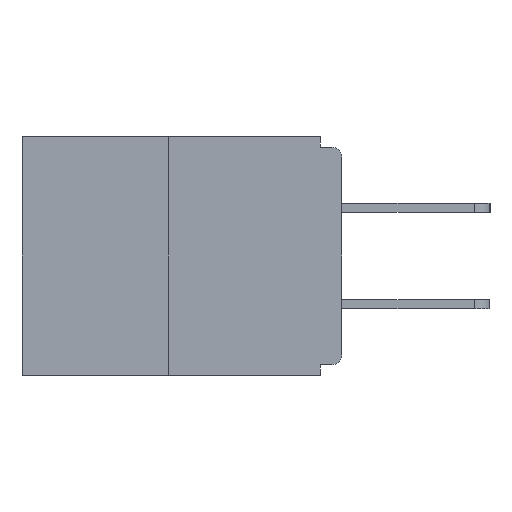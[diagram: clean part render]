
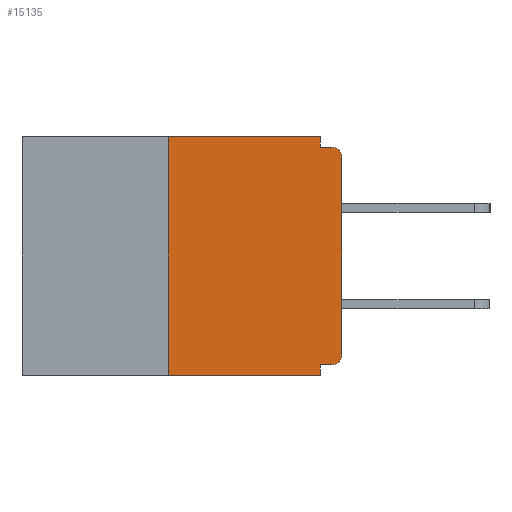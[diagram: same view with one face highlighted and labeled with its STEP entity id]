
A CAD part, left-side view. The second image highlights one B-rep face of the part: STEP entity #15135.
In plain terms, the highlighted planar face has unit normal (-1, 0, 0).
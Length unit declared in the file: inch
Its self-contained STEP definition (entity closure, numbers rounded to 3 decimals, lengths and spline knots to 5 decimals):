
#8 = CARTESIAN_POINT ( 'NONE',  ( 0., 0.015, -0.015 ) ) ;
#1059 = CARTESIAN_POINT ( 'NONE',  ( 0., 0.015, -0.03 ) ) ;
#1124 = CARTESIAN_POINT ( 'NONE',  ( 0., 0.015, -0.313 ) ) ;
#1439 = CARTESIAN_POINT ( 'NONE',  ( 0., 0., 0. ) ) ;
#1469 = VERTEX_POINT ( 'NONE', #16318 ) ;
#2100 = DIRECTION ( 'NONE',  ( 0., 0., -1. ) ) ;
#2277 = EDGE_LOOP ( 'NONE', ( #11711, #16246, #13082, #7259, #3381, #3264, #10527, #13912, #7482, #14920 ) ) ;
#2496 = EDGE_CURVE ( 'NONE', #3343, #14005, #4907, .T. ) ;
#2939 = LINE ( 'NONE', #13357, #13848 ) ;
#3190 = VECTOR ( 'NONE', #5323, 39.37008 ) ;
#3264 = ORIENTED_EDGE ( 'NONE', *, *, #3744, .T. ) ;
#3283 = EDGE_CURVE ( 'NONE', #13364, #11104, #16549, .T. ) ;
#3343 = VERTEX_POINT ( 'NONE', #10244 ) ;
#3381 = ORIENTED_EDGE ( 'NONE', *, *, #13331, .F. ) ;
#3552 = CARTESIAN_POINT ( 'NONE',  ( 0., 0.46, -0.343 ) ) ;
#3625 = DIRECTION ( 'NONE',  ( 0., 0., -1. ) ) ;
#3744 = EDGE_CURVE ( 'NONE', #7836, #12753, #15659, .T. ) ;
#3827 = CARTESIAN_POINT ( 'NONE',  ( 0., 0.25, 0. ) ) ;
#3950 = VECTOR ( 'NONE', #2100, 39.37008 ) ;
#4177 = CARTESIAN_POINT ( 'NONE',  ( 0., 0.031, 0. ) ) ;
#4307 = LINE ( 'NONE', #3827, #13775 ) ;
#4898 = EDGE_CURVE ( 'NONE', #14005, #1469, #12916, .T. ) ;
#4907 = LINE ( 'NONE', #15378, #3190 ) ;
#4911 = DIRECTION ( 'NONE',  ( 0., 0., -1. ) ) ;
#5025 = DIRECTION ( 'NONE',  ( 0., 0., -1. ) ) ;
#5040 = CARTESIAN_POINT ( 'NONE',  ( 0., 0.015, -0.328 ) ) ;
#5323 = DIRECTION ( 'NONE',  ( 0., -1., 0. ) ) ;
#5356 = EDGE_CURVE ( 'NONE', #1469, #11104, #10057, .T. ) ;
#6142 = DIRECTION ( 'NONE',  ( 0., 0., -1. ) ) ;
#7107 = VECTOR ( 'NONE', #8854, 39.37008 ) ;
#7134 = AXIS2_PLACEMENT_3D ( 'NONE', #1059, #15406, #5025 ) ;
#7259 = ORIENTED_EDGE ( 'NONE', *, *, #13041, .F. ) ;
#7337 = CARTESIAN_POINT ( 'NONE',  ( 0., 0.031, -0.343 ) ) ;
#7424 = DIRECTION ( 'NONE',  ( 0., -1., 0. ) ) ;
#7482 = ORIENTED_EDGE ( 'NONE', *, *, #5356, .F. ) ;
#7490 = VECTOR ( 'NONE', #10809, 39.37008 ) ;
#7836 = VERTEX_POINT ( 'NONE', #5040 ) ;
#8184 = DIRECTION ( 'NONE',  ( 0., 1., 0. ) ) ;
#8222 = VERTEX_POINT ( 'NONE', #7337 ) ;
#8263 = EDGE_CURVE ( 'NONE', #11462, #8222, #11537, .T. ) ;
#8276 = DIRECTION ( 'NONE',  ( 0., 0., 1. ) ) ;
#8436 = CARTESIAN_POINT ( 'NONE',  ( 0., 0., -0.03 ) ) ;
#8791 = CARTESIAN_POINT ( 'NONE',  ( 0., 0.031, -0.343 ) ) ;
#8854 = DIRECTION ( 'NONE',  ( 0., -1., 0. ) ) ;
#8973 = CARTESIAN_POINT ( 'NONE',  ( 0., 0., -0.313 ) ) ;
#9535 = VECTOR ( 'NONE', #6142, 39.37008 ) ;
#10057 = LINE ( 'NONE', #14184, #7107 ) ;
#10244 = CARTESIAN_POINT ( 'NONE',  ( 0., 0.25, 0. ) ) ;
#10247 = CARTESIAN_POINT ( 'NONE',  ( 0., 0.031, 0. ) ) ;
#10460 = EDGE_CURVE ( 'NONE', #11462, #3343, #4307, .T. ) ;
#10527 = ORIENTED_EDGE ( 'NONE', *, *, #11325, .T. ) ;
#10809 = DIRECTION ( 'NONE',  ( 0., 0., 1. ) ) ;
#11104 = VERTEX_POINT ( 'NONE', #8 ) ;
#11325 = EDGE_CURVE ( 'NONE', #12753, #13364, #11992, .T. ) ;
#11446 = DIRECTION ( 'NONE',  ( 1., 0., 0. ) ) ;
#11462 = VERTEX_POINT ( 'NONE', #12348 ) ;
#11537 = LINE ( 'NONE', #3552, #14043 ) ;
#11711 = ORIENTED_EDGE ( 'NONE', *, *, #2496, .F. ) ;
#11992 = LINE ( 'NONE', #1439, #7490 ) ;
#12348 = CARTESIAN_POINT ( 'NONE',  ( 0., 0.25, -0.343 ) ) ;
#12681 = LINE ( 'NONE', #8791, #3950 ) ;
#12753 = VERTEX_POINT ( 'NONE', #8973 ) ;
#12916 = LINE ( 'NONE', #10247, #9535 ) ;
#13041 = EDGE_CURVE ( 'NONE', #15064, #8222, #12681, .T. ) ;
#13082 = ORIENTED_EDGE ( 'NONE', *, *, #8263, .T. ) ;
#13331 = EDGE_CURVE ( 'NONE', #7836, #15064, #2939, .T. ) ;
#13357 = CARTESIAN_POINT ( 'NONE',  ( 0., 0., -0.328 ) ) ;
#13364 = VERTEX_POINT ( 'NONE', #8436 ) ;
#13775 = VECTOR ( 'NONE', #8276, 39.37008 ) ;
#13848 = VECTOR ( 'NONE', #8184, 39.37008 ) ;
#13912 = ORIENTED_EDGE ( 'NONE', *, *, #3283, .T. ) ;
#14005 = VERTEX_POINT ( 'NONE', #4177 ) ;
#14031 = PLANE ( 'NONE',  #16162 ) ;
#14043 = VECTOR ( 'NONE', #7424, 39.37008 ) ;
#14184 = CARTESIAN_POINT ( 'NONE',  ( 0., 0., -0.015 ) ) ;
#14790 = CARTESIAN_POINT ( 'NONE',  ( 0., 0.031, -0.328 ) ) ;
#14831 = AXIS2_PLACEMENT_3D ( 'NONE', #1124, #16692, #4911 ) ;
#14920 = ORIENTED_EDGE ( 'NONE', *, *, #4898, .F. ) ;
#14965 = FACE_OUTER_BOUND ( 'NONE', #2277, .T. ) ;
#15064 = VERTEX_POINT ( 'NONE', #14790 ) ;
#15135 = ADVANCED_FACE ( 'NONE', ( #14965 ), #14031, .F. ) ;
#15302 = CARTESIAN_POINT ( 'NONE',  ( 0., 0.46, 0. ) ) ;
#15378 = CARTESIAN_POINT ( 'NONE',  ( 0., 0.46, 0. ) ) ;
#15406 = DIRECTION ( 'NONE',  ( -1., 0., 0. ) ) ;
#15659 = CIRCLE ( 'NONE', #14831, 0.015 ) ;
#16162 = AXIS2_PLACEMENT_3D ( 'NONE', #15302, #11446, #3625 ) ;
#16246 = ORIENTED_EDGE ( 'NONE', *, *, #10460, .F. ) ;
#16318 = CARTESIAN_POINT ( 'NONE',  ( 0., 0.031, -0.015 ) ) ;
#16549 = CIRCLE ( 'NONE', #7134, 0.015 ) ;
#16692 = DIRECTION ( 'NONE',  ( -1., 0., 0. ) ) ;
